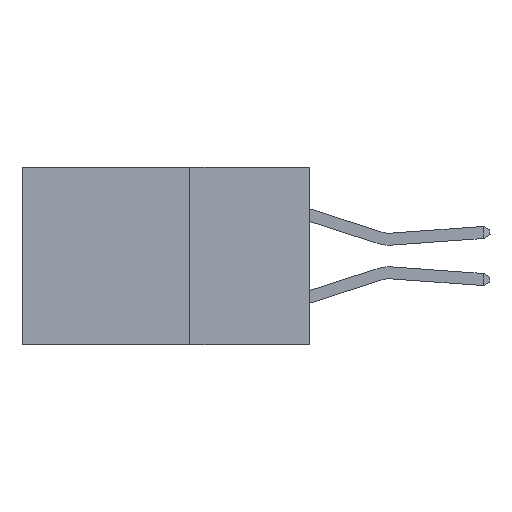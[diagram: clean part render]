
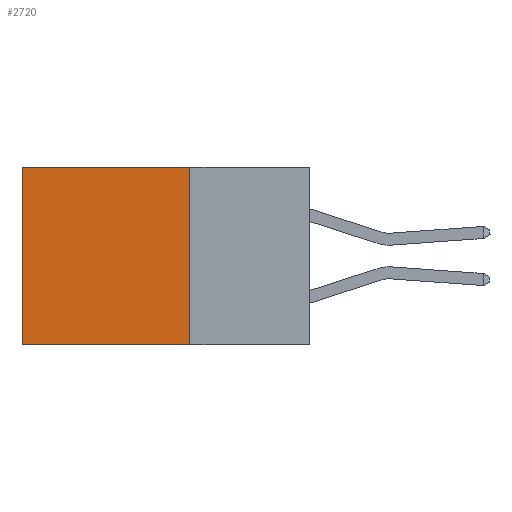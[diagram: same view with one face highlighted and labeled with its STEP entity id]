
A CAD part, left-side view. The second image highlights one B-rep face of the part: STEP entity #2720.
In plain terms, the highlighted planar face has unit normal (-1, 0, 0).
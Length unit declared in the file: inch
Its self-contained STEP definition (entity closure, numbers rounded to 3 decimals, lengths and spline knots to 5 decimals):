
#756 = ORIENTED_EDGE ( 'NONE', *, *, #7488, .T. ) ;
#1537 = EDGE_CURVE ( 'NONE', #5666, #7784, #9978, .T. ) ;
#1730 = EDGE_CURVE ( 'NONE', #9449, #13792, #12694, .T. ) ;
#2162 = ORIENTED_EDGE ( 'NONE', *, *, #1730, .T. ) ;
#2720 = ADVANCED_FACE ( 'NONE', ( #12354 ), #13640, .F. ) ;
#3030 = EDGE_LOOP ( 'NONE', ( #756, #10098, #12965, #2162 ) ) ;
#4515 = LINE ( 'NONE', #10097, #6769 ) ;
#5562 = CARTESIAN_POINT ( 'NONE',  ( 0.2615, 0.6, -0.37 ) ) ;
#5666 = VERTEX_POINT ( 'NONE', #11854 ) ;
#5968 = CARTESIAN_POINT ( 'NONE',  ( 0.2615, 0.6, 0. ) ) ;
#6066 = CARTESIAN_POINT ( 'NONE',  ( 0.2615, 0.25, -0.37 ) ) ;
#6769 = VECTOR ( 'NONE', #12572, 39.37008 ) ;
#7161 = VECTOR ( 'NONE', #9047, 39.37008 ) ;
#7203 = CARTESIAN_POINT ( 'NONE',  ( 0.2615, 0.25, 0. ) ) ;
#7488 = EDGE_CURVE ( 'NONE', #13792, #7784, #13617, .T. ) ;
#7784 = VERTEX_POINT ( 'NONE', #5562 ) ;
#9047 = DIRECTION ( 'NONE',  ( 0., 0., -1. ) ) ;
#9113 = CARTESIAN_POINT ( 'NONE',  ( 0.2615, 0.6, -0.37 ) ) ;
#9292 = EDGE_CURVE ( 'NONE', #9449, #5666, #4515, .T. ) ;
#9449 = VERTEX_POINT ( 'NONE', #9950 ) ;
#9880 = DIRECTION ( 'NONE',  ( 0., 1., 0. ) ) ;
#9950 = CARTESIAN_POINT ( 'NONE',  ( 0.2615, 0.25, 0. ) ) ;
#9978 = LINE ( 'NONE', #6066, #13176 ) ;
#10097 = CARTESIAN_POINT ( 'NONE',  ( 0.2615, 0.25, -0.37 ) ) ;
#10098 = ORIENTED_EDGE ( 'NONE', *, *, #1537, .F. ) ;
#10161 = AXIS2_PLACEMENT_3D ( 'NONE', #13873, #13615, #12111 ) ;
#11854 = CARTESIAN_POINT ( 'NONE',  ( 0.2615, 0.25, -0.37 ) ) ;
#12111 = DIRECTION ( 'NONE',  ( 0., 0., -1. ) ) ;
#12354 = FACE_OUTER_BOUND ( 'NONE', #3030, .T. ) ;
#12572 = DIRECTION ( 'NONE',  ( 0., 0., -1. ) ) ;
#12694 = LINE ( 'NONE', #7203, #13010 ) ;
#12965 = ORIENTED_EDGE ( 'NONE', *, *, #9292, .F. ) ;
#13010 = VECTOR ( 'NONE', #13672, 39.37008 ) ;
#13176 = VECTOR ( 'NONE', #9880, 39.37008 ) ;
#13615 = DIRECTION ( 'NONE',  ( 1., 0., 0. ) ) ;
#13617 = LINE ( 'NONE', #9113, #7161 ) ;
#13640 = PLANE ( 'NONE',  #10161 ) ;
#13672 = DIRECTION ( 'NONE',  ( 0., 1., 0. ) ) ;
#13792 = VERTEX_POINT ( 'NONE', #5968 ) ;
#13873 = CARTESIAN_POINT ( 'NONE',  ( 0.2615, 0.25, -0.37 ) ) ;
